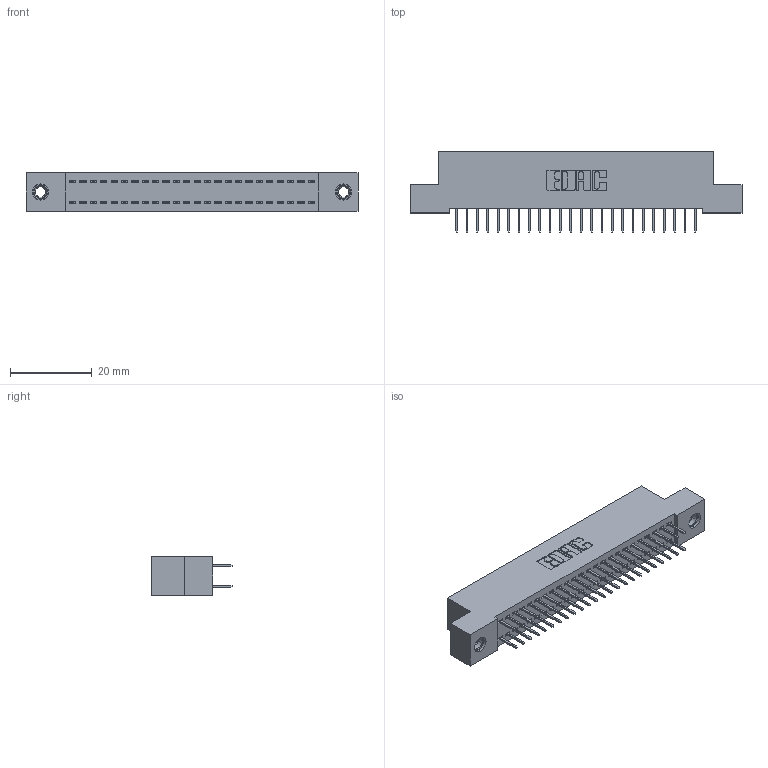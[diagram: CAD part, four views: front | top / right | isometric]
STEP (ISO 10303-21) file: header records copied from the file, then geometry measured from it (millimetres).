
FILE_DESCRIPTION (( 'STEP AP203' ), '1' );
FILE_NAME ('392-048-524-207.STEP', '2019-10-08T00:59:09', ( '' ), ( '' ), 'SwSTEP 2.0', 'SolidWorks 2016', '' );
FILE_SCHEMA (( 'CONFIG_CONTROL_DESIGN' ));
Length unit declared in the file: inch
Products named in the file (4): 345-292-001_345-293-124; 345-250-001_345-250-005-103; 392-048-524-207; 342 Part_TI
Assembly tree (51 placements, depth 2):
  392-048-524-207
    342 Part_TI
    345-292-001_345-293-124  x48
    345-250-001_345-250-005-103  x2
Bounding box: 81.28 x 19.69 x 9.4 mm (x, y, z)
Volume: 7132.5 mm3; surface area: 11003.2 mm2
Topology: 51 solids, 51 shells, 2858 faces, 8067 edges, 5178 vertices
Faces by surface type: plane 2114, cylinder 728, cone 12, torus 4
Entity records: 18896 total; most frequent: CARTESIAN_POINT 3133, ORIENTED_EDGE 3062, DIRECTION 2741, EDGE_CURVE 1531, LINE 1387, VECTOR 1387, VERTEX_POINT 1012, AXIS2_PLACEMENT_3D 677
